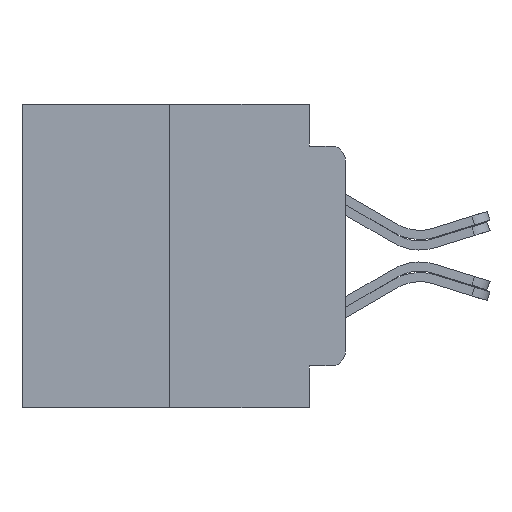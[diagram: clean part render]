
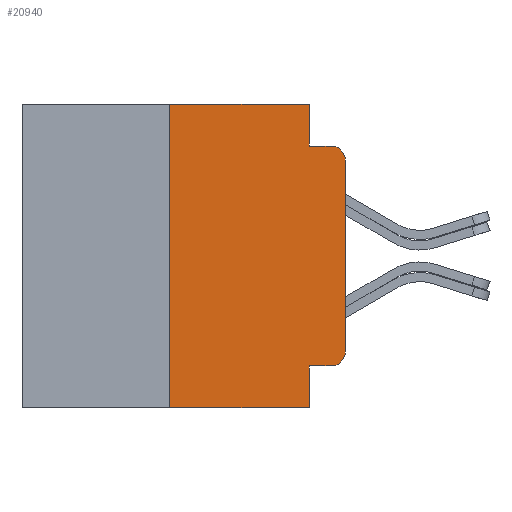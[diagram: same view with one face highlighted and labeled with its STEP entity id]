
A CAD part, left-side view. The second image highlights one B-rep face of the part: STEP entity #20940.
In plain terms, the highlighted planar face has unit normal (-1, 0, 0).
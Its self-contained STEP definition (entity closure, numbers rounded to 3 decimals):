
#363 = CARTESIAN_POINT ( 'NONE',  ( -75.603, 6.35, 5.486 ) ) ;
#443 = ORIENTED_EDGE ( 'NONE', *, *, #19321, .F. ) ;
#550 = EDGE_CURVE ( 'NONE', #25998, #18552, #5712, .T. ) ;
#776 = VERTEX_POINT ( 'NONE', #9327 ) ;
#1340 = ORIENTED_EDGE ( 'NONE', *, *, #24922, .T. ) ;
#2440 = DIRECTION ( 'NONE',  ( 0., 0., -1. ) ) ;
#2528 = PLANE ( 'NONE',  #12878 ) ;
#2662 = CARTESIAN_POINT ( 'NONE',  ( -75.603, 0.508, -3.467 ) ) ;
#2784 = ORIENTED_EDGE ( 'NONE', *, *, #22201, .T. ) ;
#3228 = CARTESIAN_POINT ( 'NONE',  ( -75.603, 11.684, 5.486 ) ) ;
#4233 = CARTESIAN_POINT ( 'NONE',  ( -75.603, 0., -3.467 ) ) ;
#4328 = CARTESIAN_POINT ( 'NONE',  ( -75.603, 1.295, -3.975 ) ) ;
#4390 = CARTESIAN_POINT ( 'NONE',  ( -75.603, 6.35, -5.486 ) ) ;
#4844 = CARTESIAN_POINT ( 'NONE',  ( -75.603, 1.295, 0. ) ) ;
#5323 = CARTESIAN_POINT ( 'NONE',  ( -75.603, 11.684, -5.486 ) ) ;
#5712 = LINE ( 'NONE', #13655, #16567 ) ;
#5762 = VERTEX_POINT ( 'NONE', #29840 ) ;
#5849 = ORIENTED_EDGE ( 'NONE', *, *, #21526, .T. ) ;
#7129 = LINE ( 'NONE', #3228, #12540 ) ;
#7644 = DIRECTION ( 'NONE',  ( 0., -1., 0. ) ) ;
#7721 = DIRECTION ( 'NONE',  ( 0., 0., -1. ) ) ;
#8050 = VECTOR ( 'NONE', #7644, 1000. ) ;
#8386 = LINE ( 'NONE', #5323, #8050 ) ;
#9291 = AXIS2_PLACEMENT_3D ( 'NONE', #21583, #24055, #7721 ) ;
#9327 = CARTESIAN_POINT ( 'NONE',  ( -75.603, 0.508, -3.975 ) ) ;
#9536 = LINE ( 'NONE', #4844, #20389 ) ;
#9893 = EDGE_CURVE ( 'NONE', #13877, #776, #11496, .T. ) ;
#9998 = EDGE_CURVE ( 'NONE', #29506, #17239, #10747, .T. ) ;
#10747 = LINE ( 'NONE', #4390, #17951 ) ;
#10844 = VECTOR ( 'NONE', #12694, 1000. ) ;
#11222 = VECTOR ( 'NONE', #11556, 1000. ) ;
#11496 = LINE ( 'NONE', #24680, #25922 ) ;
#11556 = DIRECTION ( 'NONE',  ( 0., 0., 1. ) ) ;
#11669 = EDGE_CURVE ( 'NONE', #18552, #5762, #28459, .T. ) ;
#12540 = VECTOR ( 'NONE', #23892, 1000. ) ;
#12694 = DIRECTION ( 'NONE',  ( 0., -1., 0. ) ) ;
#12878 = AXIS2_PLACEMENT_3D ( 'NONE', #16067, #21013, #18371 ) ;
#13655 = CARTESIAN_POINT ( 'NONE',  ( -75.603, 1.295, 0. ) ) ;
#13877 = VERTEX_POINT ( 'NONE', #4328 ) ;
#14227 = EDGE_LOOP ( 'NONE', ( #18437, #5849, #17388, #1340, #23698, #15238, #443, #20129, #2784, #25612 ) ) ;
#15238 = ORIENTED_EDGE ( 'NONE', *, *, #550, .F. ) ;
#15663 = DIRECTION ( 'NONE',  ( 0., 0., -1. ) ) ;
#16067 = CARTESIAN_POINT ( 'NONE',  ( -75.603, 11.684, 5.486 ) ) ;
#16428 = VERTEX_POINT ( 'NONE', #22606 ) ;
#16567 = VECTOR ( 'NONE', #15663, 1000. ) ;
#17239 = VERTEX_POINT ( 'NONE', #363 ) ;
#17388 = ORIENTED_EDGE ( 'NONE', *, *, #24617, .T. ) ;
#17417 = DIRECTION ( 'NONE',  ( 0., -1., 0. ) ) ;
#17625 = CARTESIAN_POINT ( 'NONE',  ( -75.603, 0., 3.467 ) ) ;
#17951 = VECTOR ( 'NONE', #27291, 1000. ) ;
#18371 = DIRECTION ( 'NONE',  ( 0., 0., -1. ) ) ;
#18437 = ORIENTED_EDGE ( 'NONE', *, *, #9893, .T. ) ;
#18552 = VERTEX_POINT ( 'NONE', #25814 ) ;
#19321 = EDGE_CURVE ( 'NONE', #17239, #25998, #7129, .T. ) ;
#19590 = VERTEX_POINT ( 'NONE', #17625 ) ;
#20129 = ORIENTED_EDGE ( 'NONE', *, *, #9998, .F. ) ;
#20389 = VECTOR ( 'NONE', #2440, 1000. ) ;
#20445 = FACE_OUTER_BOUND ( 'NONE', #14227, .T. ) ;
#20940 = ADVANCED_FACE ( 'NONE', ( #20445 ), #2528, .F. ) ;
#20989 = LINE ( 'NONE', #27687, #11222 ) ;
#21013 = DIRECTION ( 'NONE',  ( 1., 0., 0. ) ) ;
#21526 = EDGE_CURVE ( 'NONE', #776, #23699, #27591, .T. ) ;
#21583 = CARTESIAN_POINT ( 'NONE',  ( -75.603, 0.508, 3.467 ) ) ;
#22201 = EDGE_CURVE ( 'NONE', #29506, #16428, #8386, .T. ) ;
#22606 = CARTESIAN_POINT ( 'NONE',  ( -75.603, 1.295, -5.486 ) ) ;
#22807 = CARTESIAN_POINT ( 'NONE',  ( -75.603, 1.295, 5.486 ) ) ;
#23222 = DIRECTION ( 'NONE',  ( -1., 0., 0. ) ) ;
#23698 = ORIENTED_EDGE ( 'NONE', *, *, #11669, .F. ) ;
#23699 = VERTEX_POINT ( 'NONE', #4233 ) ;
#23892 = DIRECTION ( 'NONE',  ( 0., -1., 0. ) ) ;
#24055 = DIRECTION ( 'NONE',  ( -1., 0., 0. ) ) ;
#24617 = EDGE_CURVE ( 'NONE', #23699, #19590, #20989, .T. ) ;
#24680 = CARTESIAN_POINT ( 'NONE',  ( -75.603, 1.295, -3.975 ) ) ;
#24922 = EDGE_CURVE ( 'NONE', #19590, #5762, #28515, .T. ) ;
#25468 = DIRECTION ( 'NONE',  ( 0., 0., -1. ) ) ;
#25612 = ORIENTED_EDGE ( 'NONE', *, *, #29246, .F. ) ;
#25814 = CARTESIAN_POINT ( 'NONE',  ( -75.603, 1.295, 3.975 ) ) ;
#25922 = VECTOR ( 'NONE', #17417, 1000. ) ;
#25998 = VERTEX_POINT ( 'NONE', #22807 ) ;
#26616 = CARTESIAN_POINT ( 'NONE',  ( -75.603, 1.295, 3.975 ) ) ;
#27291 = DIRECTION ( 'NONE',  ( 0., 0., 1. ) ) ;
#27591 = CIRCLE ( 'NONE', #28318, 0.508 ) ;
#27687 = CARTESIAN_POINT ( 'NONE',  ( -75.603, 0., 5.486 ) ) ;
#28222 = CARTESIAN_POINT ( 'NONE',  ( -75.603, 6.35, -5.486 ) ) ;
#28318 = AXIS2_PLACEMENT_3D ( 'NONE', #2662, #23222, #25468 ) ;
#28459 = LINE ( 'NONE', #26616, #10844 ) ;
#28515 = CIRCLE ( 'NONE', #9291, 0.508 ) ;
#29246 = EDGE_CURVE ( 'NONE', #13877, #16428, #9536, .T. ) ;
#29506 = VERTEX_POINT ( 'NONE', #28222 ) ;
#29840 = CARTESIAN_POINT ( 'NONE',  ( -75.603, 0.508, 3.975 ) ) ;
